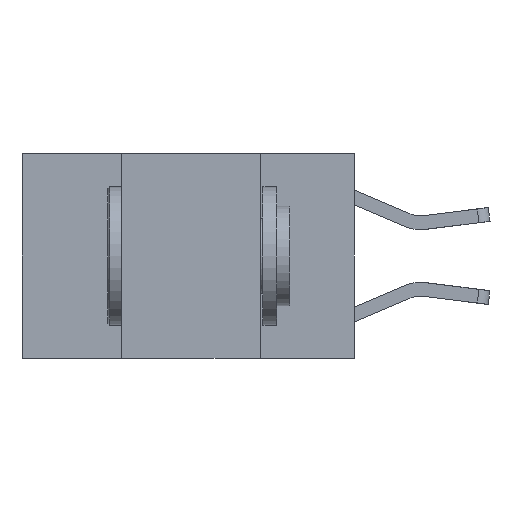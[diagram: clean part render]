
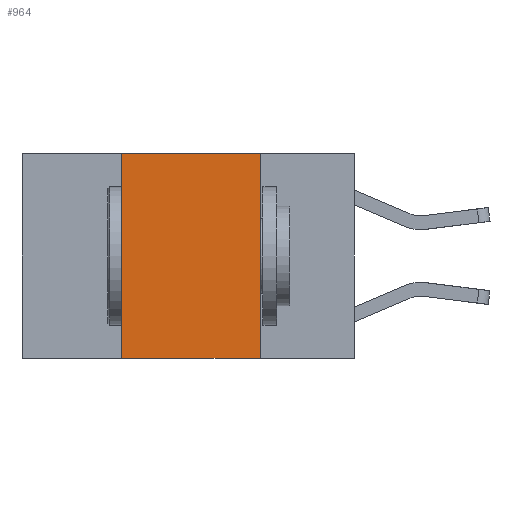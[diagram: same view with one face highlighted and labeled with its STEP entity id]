
A CAD part, left-side view. The second image highlights one B-rep face of the part: STEP entity #964.
In plain terms, the highlighted planar face has unit normal (-1, 0, 0).
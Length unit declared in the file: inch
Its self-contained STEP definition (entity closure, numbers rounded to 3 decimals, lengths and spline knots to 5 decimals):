
#776 = VERTEX_POINT ( 'NONE', #4275 ) ;
#882 = VECTOR ( 'NONE', #4272, 39.37008 ) ;
#964 = ADVANCED_FACE ( 'NONE', ( #5898 ), #6802, .F. ) ;
#1785 = DIRECTION ( 'NONE',  ( 0., -1., 0. ) ) ;
#1885 = LINE ( 'NONE', #1894, #10178 ) ;
#1894 = CARTESIAN_POINT ( 'NONE',  ( 0., 0.6, -0.37 ) ) ;
#2224 = DIRECTION ( 'NONE',  ( 0., 0., -1. ) ) ;
#2841 = VECTOR ( 'NONE', #3832, 39.37008 ) ;
#3073 = EDGE_CURVE ( 'NONE', #8329, #776, #1885, .T. ) ;
#3452 = CARTESIAN_POINT ( 'NONE',  ( 0., 0.42, 0. ) ) ;
#3832 = DIRECTION ( 'NONE',  ( 0., 0., -1. ) ) ;
#4081 = VERTEX_POINT ( 'NONE', #7953 ) ;
#4272 = DIRECTION ( 'NONE',  ( 0., 0., 1. ) ) ;
#4275 = CARTESIAN_POINT ( 'NONE',  ( 0., 0.17, -0.37 ) ) ;
#4929 = ORIENTED_EDGE ( 'NONE', *, *, #8862, .F. ) ;
#5006 = LINE ( 'NONE', #10161, #2841 ) ;
#5662 = DIRECTION ( 'NONE',  ( 0., -1., 0. ) ) ;
#5689 = ORIENTED_EDGE ( 'NONE', *, *, #7943, .F. ) ;
#5898 = FACE_OUTER_BOUND ( 'NONE', #8415, .T. ) ;
#5938 = ORIENTED_EDGE ( 'NONE', *, *, #3073, .T. ) ;
#6175 = AXIS2_PLACEMENT_3D ( 'NONE', #8196, #9353, #2224 ) ;
#6500 = CARTESIAN_POINT ( 'NONE',  ( 0., 0.17, 0. ) ) ;
#6553 = VECTOR ( 'NONE', #5662, 39.37008 ) ;
#6802 = PLANE ( 'NONE',  #6175 ) ;
#7071 = ORIENTED_EDGE ( 'NONE', *, *, #7800, .F. ) ;
#7432 = LINE ( 'NONE', #3452, #882 ) ;
#7800 = EDGE_CURVE ( 'NONE', #4081, #8463, #8422, .T. ) ;
#7943 = EDGE_CURVE ( 'NONE', #8329, #4081, #7432, .T. ) ;
#7953 = CARTESIAN_POINT ( 'NONE',  ( 0., 0.42, 0. ) ) ;
#8196 = CARTESIAN_POINT ( 'NONE',  ( 0., 0.6, 0. ) ) ;
#8329 = VERTEX_POINT ( 'NONE', #10259 ) ;
#8415 = EDGE_LOOP ( 'NONE', ( #4929, #7071, #5689, #5938 ) ) ;
#8422 = LINE ( 'NONE', #10365, #6553 ) ;
#8463 = VERTEX_POINT ( 'NONE', #6500 ) ;
#8862 = EDGE_CURVE ( 'NONE', #8463, #776, #5006, .T. ) ;
#9353 = DIRECTION ( 'NONE',  ( 1., 0., 0. ) ) ;
#10161 = CARTESIAN_POINT ( 'NONE',  ( 0., 0.17, 0. ) ) ;
#10178 = VECTOR ( 'NONE', #1785, 39.37008 ) ;
#10259 = CARTESIAN_POINT ( 'NONE',  ( 0., 0.42, -0.37 ) ) ;
#10365 = CARTESIAN_POINT ( 'NONE',  ( 0., 0.6, 0. ) ) ;
